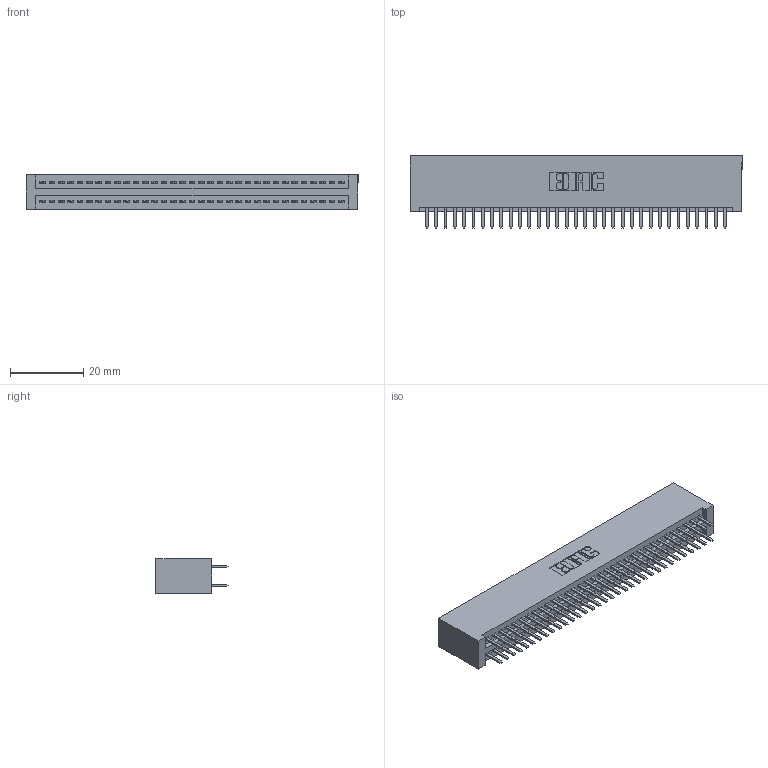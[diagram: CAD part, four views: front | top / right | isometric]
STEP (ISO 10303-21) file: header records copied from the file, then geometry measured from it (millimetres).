
FILE_DESCRIPTION (( 'STEP AP203' ), '1' );
FILE_NAME ('395-066-520-201.STEP', '2018-11-25T00:26:24', ( '' ), ( '' ), 'SwSTEP 2.0', 'SolidWorks 2016', '' );
FILE_SCHEMA (( 'CONFIG_CONTROL_DESIGN' ));
Length unit declared in the file: inch
Products named in the file (3): 395-066-520-201; 345-292-001_345-293-120; 345 Part_No Mounting Lugs
Assembly tree (67 placements, depth 2):
  395-066-520-201
    345 Part_No Mounting Lugs
    345-292-001_345-293-120  x66
Bounding box: 90.42 x 19.68 x 9.4 mm (x, y, z)
Volume: 9287.2 mm3; surface area: 13795.3 mm2
Topology: 67 solids, 67 shells, 3682 faces, 10679 edges, 6942 vertices
Faces by surface type: plane 2386, cylinder 1296
Entity records: 26941 total; most frequent: CARTESIAN_POINT 4536, ORIENTED_EDGE 4458, DIRECTION 3993, EDGE_CURVE 2229, VECTOR 1969, LINE 1969, VERTEX_POINT 1482, AXIS2_PLACEMENT_3D 1012
